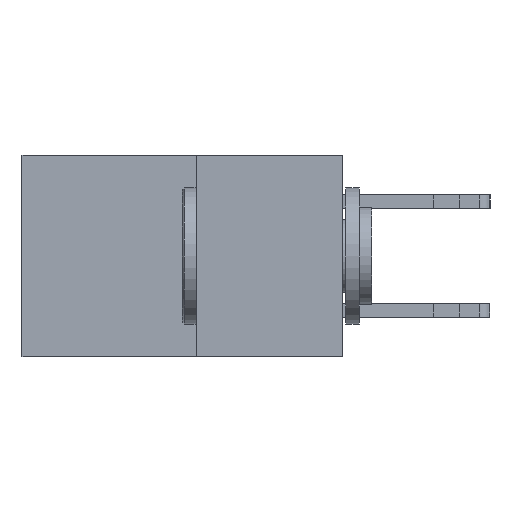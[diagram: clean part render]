
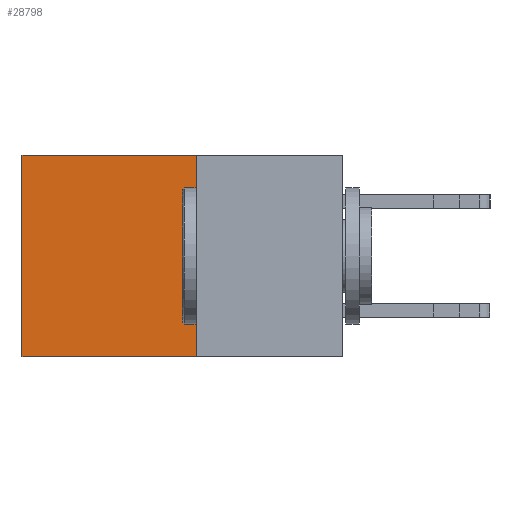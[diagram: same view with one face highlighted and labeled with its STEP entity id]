
A CAD part, left-side view. The second image highlights one B-rep face of the part: STEP entity #28798.
In plain terms, the highlighted planar face has unit normal (-1, 0, 0).
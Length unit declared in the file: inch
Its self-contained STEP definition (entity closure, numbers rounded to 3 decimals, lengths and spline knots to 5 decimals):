
#359 = ORIENTED_EDGE ( 'NONE', *, *, #1004, .F. ) ;
#443 = VECTOR ( 'NONE', #10090, 39.37008 ) ;
#873 = CARTESIAN_POINT ( 'NONE',  ( 0.277, 0.27, 0. ) ) ;
#1004 = EDGE_CURVE ( 'NONE', #22278, #5861, #12869, .T. ) ;
#1320 = CARTESIAN_POINT ( 'NONE',  ( 0.277, 0.27, -0.37 ) ) ;
#3662 = VECTOR ( 'NONE', #20554, 39.37008 ) ;
#3895 = DIRECTION ( 'NONE',  ( 0., 0., -1. ) ) ;
#5861 = VERTEX_POINT ( 'NONE', #9398 ) ;
#6273 = ORIENTED_EDGE ( 'NONE', *, *, #14806, .T. ) ;
#7381 = CARTESIAN_POINT ( 'NONE',  ( 0.277, 0.59, 0. ) ) ;
#8968 = VECTOR ( 'NONE', #13576, 39.37008 ) ;
#9213 = CARTESIAN_POINT ( 'NONE',  ( 0.277, 0.27, -0.37 ) ) ;
#9398 = CARTESIAN_POINT ( 'NONE',  ( 0.277, 0.59, -0.37 ) ) ;
#10090 = DIRECTION ( 'NONE',  ( 0., 0., -1. ) ) ;
#11021 = CARTESIAN_POINT ( 'NONE',  ( 0.277, 0.27, -0.37 ) ) ;
#12513 = EDGE_LOOP ( 'NONE', ( #27145, #359, #19414, #6273 ) ) ;
#12869 = LINE ( 'NONE', #31937, #25358 ) ;
#13153 = CARTESIAN_POINT ( 'NONE',  ( 0.277, 0.59, -0.37 ) ) ;
#13576 = DIRECTION ( 'NONE',  ( 0., 0., -1. ) ) ;
#13976 = PLANE ( 'NONE',  #19090 ) ;
#14806 = EDGE_CURVE ( 'NONE', #29055, #23752, #30469, .T. ) ;
#14849 = FACE_OUTER_BOUND ( 'NONE', #12513, .T. ) ;
#15563 = CARTESIAN_POINT ( 'NONE',  ( 0.277, 0.27, 0. ) ) ;
#18852 = EDGE_CURVE ( 'NONE', #29055, #22278, #29049, .T. ) ;
#18983 = DIRECTION ( 'NONE',  ( 1., 0., 0. ) ) ;
#19090 = AXIS2_PLACEMENT_3D ( 'NONE', #1320, #18983, #3895 ) ;
#19414 = ORIENTED_EDGE ( 'NONE', *, *, #18852, .F. ) ;
#20554 = DIRECTION ( 'NONE',  ( 0., 1., 0. ) ) ;
#20582 = LINE ( 'NONE', #13153, #443 ) ;
#22278 = VERTEX_POINT ( 'NONE', #9213 ) ;
#22535 = EDGE_CURVE ( 'NONE', #23752, #5861, #20582, .T. ) ;
#23752 = VERTEX_POINT ( 'NONE', #7381 ) ;
#25358 = VECTOR ( 'NONE', #31750, 39.37008 ) ;
#27145 = ORIENTED_EDGE ( 'NONE', *, *, #22535, .T. ) ;
#28798 = ADVANCED_FACE ( 'NONE', ( #14849 ), #13976, .F. ) ;
#29049 = LINE ( 'NONE', #11021, #8968 ) ;
#29055 = VERTEX_POINT ( 'NONE', #873 ) ;
#30469 = LINE ( 'NONE', #15563, #3662 ) ;
#31750 = DIRECTION ( 'NONE',  ( 0., 1., 0. ) ) ;
#31937 = CARTESIAN_POINT ( 'NONE',  ( 0.277, 0.27, -0.37 ) ) ;
